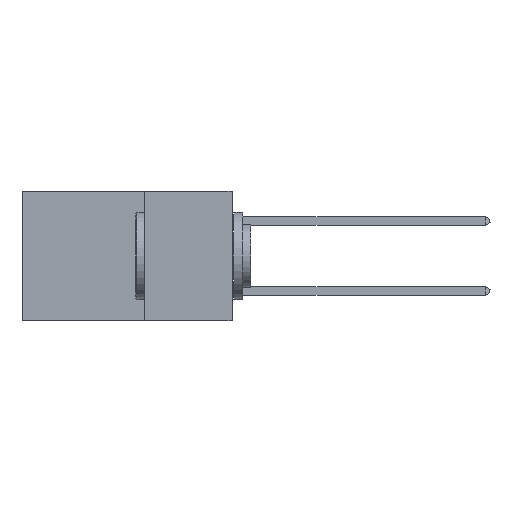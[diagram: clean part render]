
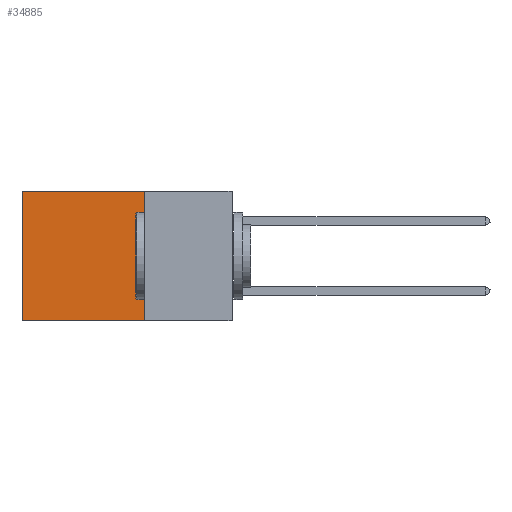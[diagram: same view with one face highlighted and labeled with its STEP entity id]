
A CAD part, left-side view. The second image highlights one B-rep face of the part: STEP entity #34885.
In plain terms, the highlighted planar face has unit normal (-1, 0, 0).
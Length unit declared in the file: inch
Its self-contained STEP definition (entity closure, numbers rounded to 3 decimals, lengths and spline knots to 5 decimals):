
#70 = DIRECTION ( 'NONE',  ( 0., 0., -1. ) ) ;
#1068 = ORIENTED_EDGE ( 'NONE', *, *, #22162, .T. ) ;
#1447 = CARTESIAN_POINT ( 'NONE',  ( 0.2875, 0.6, 0. ) ) ;
#3397 = VECTOR ( 'NONE', #23254, 39.37008 ) ;
#6771 = CARTESIAN_POINT ( 'NONE',  ( 0.2875, 0.25, 0. ) ) ;
#7411 = LINE ( 'NONE', #25116, #30188 ) ;
#9093 = VECTOR ( 'NONE', #13529, 39.37008 ) ;
#10053 = VERTEX_POINT ( 'NONE', #26019 ) ;
#10418 = CARTESIAN_POINT ( 'NONE',  ( 0.2875, 0.25, 0. ) ) ;
#11645 = VERTEX_POINT ( 'NONE', #23415 ) ;
#11727 = VERTEX_POINT ( 'NONE', #39127 ) ;
#11937 = EDGE_CURVE ( 'NONE', #35750, #11645, #38355, .T. ) ;
#13529 = DIRECTION ( 'NONE',  ( 0., 1., 0. ) ) ;
#13711 = VECTOR ( 'NONE', #70, 39.37008 ) ;
#15363 = DIRECTION ( 'NONE',  ( 0., 0., -1. ) ) ;
#18839 = DIRECTION ( 'NONE',  ( 0., 1., 0. ) ) ;
#21296 = EDGE_LOOP ( 'NONE', ( #1068, #38170, #31893, #29007 ) ) ;
#22162 = EDGE_CURVE ( 'NONE', #10053, #11727, #27200, .T. ) ;
#23254 = DIRECTION ( 'NONE',  ( 0., 0., -1. ) ) ;
#23415 = CARTESIAN_POINT ( 'NONE',  ( 0.2875, 0.25, -0.37 ) ) ;
#24469 = EDGE_CURVE ( 'NONE', #35750, #10053, #25655, .T. ) ;
#25116 = CARTESIAN_POINT ( 'NONE',  ( 0.2875, 0.25, -0.37 ) ) ;
#25655 = LINE ( 'NONE', #10418, #9093 ) ;
#26019 = CARTESIAN_POINT ( 'NONE',  ( 0.2875, 0.6, 0. ) ) ;
#27200 = LINE ( 'NONE', #1447, #3397 ) ;
#27706 = CARTESIAN_POINT ( 'NONE',  ( 0.2875, 0.25, 0. ) ) ;
#27934 = EDGE_CURVE ( 'NONE', #11645, #11727, #7411, .T. ) ;
#28251 = AXIS2_PLACEMENT_3D ( 'NONE', #27706, #33860, #15363 ) ;
#29007 = ORIENTED_EDGE ( 'NONE', *, *, #24469, .T. ) ;
#30188 = VECTOR ( 'NONE', #18839, 39.37008 ) ;
#31893 = ORIENTED_EDGE ( 'NONE', *, *, #11937, .F. ) ;
#33860 = DIRECTION ( 'NONE',  ( 1., 0., 0. ) ) ;
#34885 = ADVANCED_FACE ( 'NONE', ( #36365 ), #39928, .F. ) ;
#35750 = VERTEX_POINT ( 'NONE', #6771 ) ;
#36365 = FACE_OUTER_BOUND ( 'NONE', #21296, .T. ) ;
#37221 = CARTESIAN_POINT ( 'NONE',  ( 0.2875, 0.25, 0. ) ) ;
#38170 = ORIENTED_EDGE ( 'NONE', *, *, #27934, .F. ) ;
#38355 = LINE ( 'NONE', #37221, #13711 ) ;
#39127 = CARTESIAN_POINT ( 'NONE',  ( 0.2875, 0.6, -0.37 ) ) ;
#39928 = PLANE ( 'NONE',  #28251 ) ;
